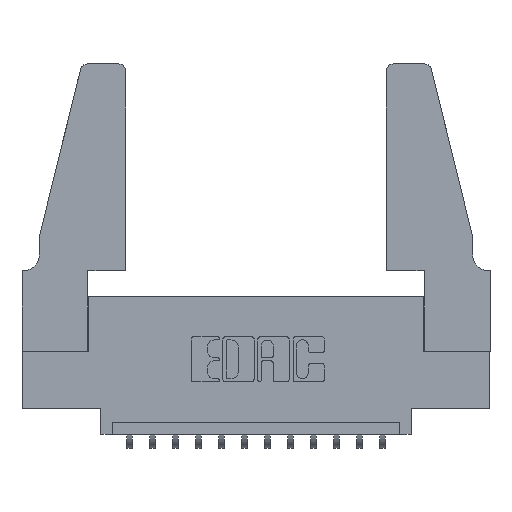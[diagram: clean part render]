
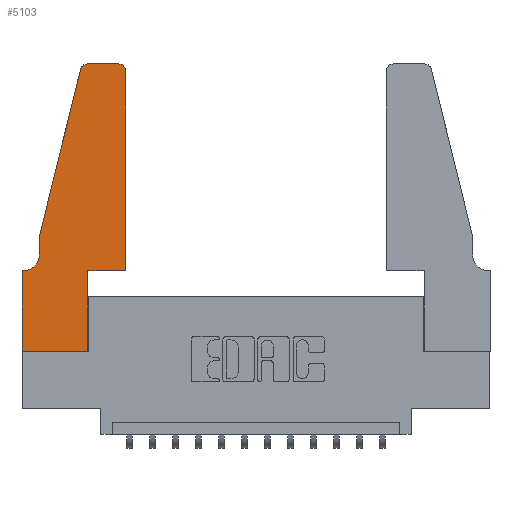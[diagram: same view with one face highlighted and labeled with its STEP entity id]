
A CAD part, top view. The second image highlights one B-rep face of the part: STEP entity #5103.
In plain terms, the highlighted planar face has unit normal (0, 0, 1).
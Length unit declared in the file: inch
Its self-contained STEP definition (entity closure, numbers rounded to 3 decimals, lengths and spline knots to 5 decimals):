
#226 = CARTESIAN_POINT ( 'NONE',  ( 0.2865, 0., 0.37 ) ) ;
#379 = AXIS2_PLACEMENT_3D ( 'NONE', #13802, #6536, #12500 ) ;
#403 = VECTOR ( 'NONE', #6290, 39.37008 ) ;
#419 = LINE ( 'NONE', #6045, #1906 ) ;
#614 = LINE ( 'NONE', #14710, #14397 ) ;
#642 = ORIENTED_EDGE ( 'NONE', *, *, #7846, .T. ) ;
#765 = CARTESIAN_POINT ( 'NONE',  ( 0., 0., 0.37 ) ) ;
#1184 = LINE ( 'NONE', #9437, #13504 ) ;
#1455 = CARTESIAN_POINT ( 'NONE',  ( 0.4205, 1.22, 0.37 ) ) ;
#1906 = VECTOR ( 'NONE', #14489, 39.37008 ) ;
#1939 = VERTEX_POINT ( 'NONE', #765 ) ;
#2177 = LINE ( 'NONE', #14598, #9063 ) ;
#2230 = DIRECTION ( 'NONE',  ( 1., 0., 0. ) ) ;
#2426 = LINE ( 'NONE', #4757, #12716 ) ;
#3283 = AXIS2_PLACEMENT_3D ( 'NONE', #10707, #13211, #7148 ) ;
#3416 = EDGE_CURVE ( 'NONE', #7075, #8661, #3767, .T. ) ;
#3497 = EDGE_CURVE ( 'NONE', #12738, #7075, #614, .T. ) ;
#3502 = VERTEX_POINT ( 'NONE', #12215 ) ;
#3609 = EDGE_CURVE ( 'NONE', #11495, #5691, #1184, .T. ) ;
#3686 = EDGE_CURVE ( 'NONE', #8235, #12738, #419, .T. ) ;
#3741 = CARTESIAN_POINT ( 'NONE',  ( 0.2605, 1.25, 0.37 ) ) ;
#3767 = CIRCLE ( 'NONE', #8651, 0.07 ) ;
#3866 = VERTEX_POINT ( 'NONE', #11022 ) ;
#4666 = VERTEX_POINT ( 'NONE', #8117 ) ;
#4752 = ORIENTED_EDGE ( 'NONE', *, *, #10782, .T. ) ;
#4757 = CARTESIAN_POINT ( 'NONE',  ( 0., 0., 0.37 ) ) ;
#4766 = CARTESIAN_POINT ( 'NONE',  ( 0.4505, 1.22, 0.37 ) ) ;
#4796 = DIRECTION ( 'NONE',  ( -1., 0., 0. ) ) ;
#5103 = ADVANCED_FACE ( 'NONE', ( #7081 ), #14282, .T. ) ;
#5245 = ORIENTED_EDGE ( 'NONE', *, *, #3609, .T. ) ;
#5406 = EDGE_CURVE ( 'NONE', #1939, #11495, #2426, .T. ) ;
#5466 = LINE ( 'NONE', #6280, #14402 ) ;
#5562 = DIRECTION ( 'NONE',  ( 1., 0., 0. ) ) ;
#5691 = VERTEX_POINT ( 'NONE', #8183 ) ;
#6045 = CARTESIAN_POINT ( 'NONE',  ( 0.0755, 0.5, 0.37 ) ) ;
#6154 = CARTESIAN_POINT ( 'NONE',  ( 0.0055, 0.42, 0.37 ) ) ;
#6249 = ORIENTED_EDGE ( 'NONE', *, *, #13824, .T. ) ;
#6280 = CARTESIAN_POINT ( 'NONE',  ( 0.0755, 0.35, 0.37 ) ) ;
#6290 = DIRECTION ( 'NONE',  ( 0., 1., 0. ) ) ;
#6357 = LINE ( 'NONE', #13465, #403 ) ;
#6536 = DIRECTION ( 'NONE',  ( 0., 0., 1. ) ) ;
#6814 = CIRCLE ( 'NONE', #14117, 0.03 ) ;
#7075 = VERTEX_POINT ( 'NONE', #14745 ) ;
#7081 = FACE_OUTER_BOUND ( 'NONE', #13565, .T. ) ;
#7148 = DIRECTION ( 'NONE',  ( 1., 0., 0. ) ) ;
#7247 = LINE ( 'NONE', #3741, #13798 ) ;
#7543 = ORIENTED_EDGE ( 'NONE', *, *, #3686, .T. ) ;
#7846 = EDGE_CURVE ( 'NONE', #4666, #15355, #6357, .T. ) ;
#8117 = CARTESIAN_POINT ( 'NONE',  ( 0.4505, 0.35, 0.37 ) ) ;
#8142 = ORIENTED_EDGE ( 'NONE', *, *, #3497, .T. ) ;
#8183 = CARTESIAN_POINT ( 'NONE',  ( 0.2865, 0.35, 0.37 ) ) ;
#8235 = VERTEX_POINT ( 'NONE', #12966 ) ;
#8642 = DIRECTION ( 'NONE',  ( -1., 0., 0. ) ) ;
#8651 = AXIS2_PLACEMENT_3D ( 'NONE', #6154, #11957, #4796 ) ;
#8661 = VERTEX_POINT ( 'NONE', #11389 ) ;
#8827 = ORIENTED_EDGE ( 'NONE', *, *, #8947, .T. ) ;
#8947 = EDGE_CURVE ( 'NONE', #11992, #3866, #7247, .T. ) ;
#9063 = VECTOR ( 'NONE', #15437, 39.37008 ) ;
#9085 = ORIENTED_EDGE ( 'NONE', *, *, #12190, .T. ) ;
#9437 = CARTESIAN_POINT ( 'NONE',  ( 0.2865, 0.35, 0.37 ) ) ;
#9772 = ORIENTED_EDGE ( 'NONE', *, *, #5406, .T. ) ;
#10248 = EDGE_CURVE ( 'NONE', #3502, #1939, #2177, .T. ) ;
#10707 = CARTESIAN_POINT ( 'NONE',  ( 0., 0.35, 0.37 ) ) ;
#10782 = EDGE_CURVE ( 'NONE', #15355, #11992, #6814, .T. ) ;
#10862 = DIRECTION ( 'NONE',  ( 0., 1., 0. ) ) ;
#10872 = CARTESIAN_POINT ( 'NONE',  ( 0.0755, 0.5, 0.37 ) ) ;
#11022 = CARTESIAN_POINT ( 'NONE',  ( 0.284, 1.25, 0.37 ) ) ;
#11389 = CARTESIAN_POINT ( 'NONE',  ( 0.0055, 0.35, 0.37 ) ) ;
#11495 = VERTEX_POINT ( 'NONE', #226 ) ;
#11734 = CARTESIAN_POINT ( 'NONE',  ( 0.4505, 0.35, 0.37 ) ) ;
#11957 = DIRECTION ( 'NONE',  ( 0., 0., -1. ) ) ;
#11992 = VERTEX_POINT ( 'NONE', #14878 ) ;
#12114 = DIRECTION ( 'NONE',  ( -1., 0., 0. ) ) ;
#12190 = EDGE_CURVE ( 'NONE', #8661, #3502, #5466, .T. ) ;
#12215 = CARTESIAN_POINT ( 'NONE',  ( 0., 0.35, 0.37 ) ) ;
#12500 = DIRECTION ( 'NONE',  ( 1., 0., 0. ) ) ;
#12716 = VECTOR ( 'NONE', #2230, 39.37008 ) ;
#12738 = VERTEX_POINT ( 'NONE', #10872 ) ;
#12830 = ORIENTED_EDGE ( 'NONE', *, *, #3416, .T. ) ;
#12966 = CARTESIAN_POINT ( 'NONE',  ( 0.25487, 1.22718, 0.37 ) ) ;
#13211 = DIRECTION ( 'NONE',  ( 0., 0., 1. ) ) ;
#13465 = CARTESIAN_POINT ( 'NONE',  ( 0.4505, 0.35, 0.37 ) ) ;
#13504 = VECTOR ( 'NONE', #10862, 39.37008 ) ;
#13526 = ORIENTED_EDGE ( 'NONE', *, *, #10248, .T. ) ;
#13554 = DIRECTION ( 'NONE',  ( 0., 0., 1. ) ) ;
#13565 = EDGE_LOOP ( 'NONE', ( #8827, #14449, #7543, #8142, #12830, #9085, #13526, #9772, #5245, #6249, #642, #4752 ) ) ;
#13633 = DIRECTION ( 'NONE',  ( 0., -1., 0. ) ) ;
#13710 = EDGE_CURVE ( 'NONE', #3866, #8235, #13881, .T. ) ;
#13798 = VECTOR ( 'NONE', #8642, 39.37008 ) ;
#13802 = CARTESIAN_POINT ( 'NONE',  ( 0.284, 1.22, 0.37 ) ) ;
#13824 = EDGE_CURVE ( 'NONE', #5691, #4666, #15169, .T. ) ;
#13881 = CIRCLE ( 'NONE', #379, 0.03 ) ;
#14048 = VECTOR ( 'NONE', #5562, 39.37008 ) ;
#14117 = AXIS2_PLACEMENT_3D ( 'NONE', #1455, #13554, #14525 ) ;
#14282 = PLANE ( 'NONE',  #3283 ) ;
#14397 = VECTOR ( 'NONE', #13633, 39.37008 ) ;
#14402 = VECTOR ( 'NONE', #12114, 39.37008 ) ;
#14449 = ORIENTED_EDGE ( 'NONE', *, *, #13710, .T. ) ;
#14489 = DIRECTION ( 'NONE',  ( -0.239, -0.971, 0. ) ) ;
#14525 = DIRECTION ( 'NONE',  ( 1., 0., 0. ) ) ;
#14598 = CARTESIAN_POINT ( 'NONE',  ( 0., 0., 0.37 ) ) ;
#14710 = CARTESIAN_POINT ( 'NONE',  ( 0.0755, 0.5, 0.37 ) ) ;
#14745 = CARTESIAN_POINT ( 'NONE',  ( 0.0755, 0.42, 0.37 ) ) ;
#14878 = CARTESIAN_POINT ( 'NONE',  ( 0.4205, 1.25, 0.37 ) ) ;
#15169 = LINE ( 'NONE', #11734, #14048 ) ;
#15355 = VERTEX_POINT ( 'NONE', #4766 ) ;
#15437 = DIRECTION ( 'NONE',  ( 0., -1., 0. ) ) ;
